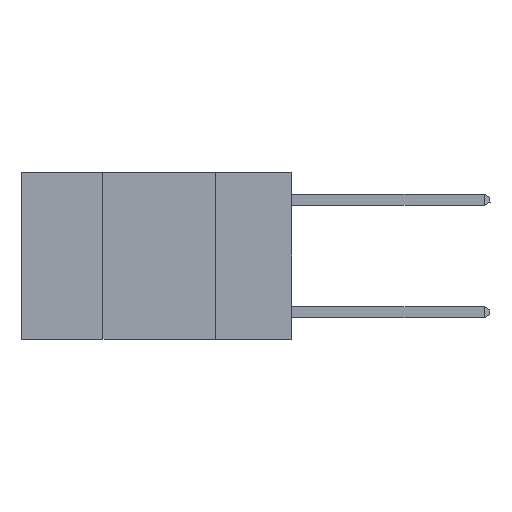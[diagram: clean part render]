
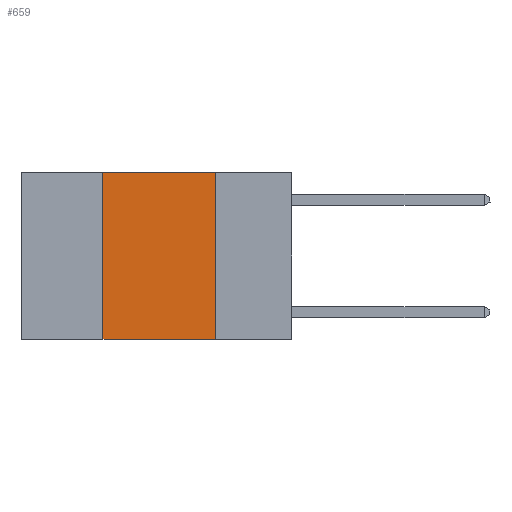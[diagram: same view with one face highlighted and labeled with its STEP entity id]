
A CAD part, left-side view. The second image highlights one B-rep face of the part: STEP entity #659.
In plain terms, the highlighted planar face has unit normal (-1, 0, 0).
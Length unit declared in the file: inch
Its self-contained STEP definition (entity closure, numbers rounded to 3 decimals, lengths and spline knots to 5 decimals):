
#45 = EDGE_LOOP ( 'NONE', ( #8960, #405, #11624, #4303 ) ) ;
#271 = VECTOR ( 'NONE', #1170, 39.37008 ) ;
#405 = ORIENTED_EDGE ( 'NONE', *, *, #2598, .F. ) ;
#479 = CARTESIAN_POINT ( 'NONE',  ( 0., 0.42, 0. ) ) ;
#531 = DIRECTION ( 'NONE',  ( 0., 0., 1. ) ) ;
#659 = ADVANCED_FACE ( 'NONE', ( #1397 ), #11835, .F. ) ;
#1170 = DIRECTION ( 'NONE',  ( 0., 0., -1. ) ) ;
#1397 = FACE_OUTER_BOUND ( 'NONE', #45, .T. ) ;
#1494 = DIRECTION ( 'NONE',  ( 0., -1., 0. ) ) ;
#1656 = CARTESIAN_POINT ( 'NONE',  ( 0., 0.6, -0.37 ) ) ;
#1747 = EDGE_CURVE ( 'NONE', #2354, #3298, #9297, .T. ) ;
#1871 = LINE ( 'NONE', #1656, #11259 ) ;
#2224 = CARTESIAN_POINT ( 'NONE',  ( 0., 0.17, -0.37 ) ) ;
#2354 = VERTEX_POINT ( 'NONE', #5978 ) ;
#2598 = EDGE_CURVE ( 'NONE', #3298, #3475, #3741, .T. ) ;
#3050 = LINE ( 'NONE', #6753, #271 ) ;
#3298 = VERTEX_POINT ( 'NONE', #8637 ) ;
#3448 = CARTESIAN_POINT ( 'NONE',  ( 0., 0.6, 0. ) ) ;
#3475 = VERTEX_POINT ( 'NONE', #5948 ) ;
#3714 = DIRECTION ( 'NONE',  ( 0., 0., -1. ) ) ;
#3741 = LINE ( 'NONE', #3955, #5592 ) ;
#3877 = DIRECTION ( 'NONE',  ( 0., -1., 0. ) ) ;
#3955 = CARTESIAN_POINT ( 'NONE',  ( 0., 0.6, 0. ) ) ;
#4303 = ORIENTED_EDGE ( 'NONE', *, *, #5254, .T. ) ;
#4455 = VECTOR ( 'NONE', #531, 39.37008 ) ;
#5254 = EDGE_CURVE ( 'NONE', #2354, #8116, #1871, .T. ) ;
#5592 = VECTOR ( 'NONE', #3877, 39.37008 ) ;
#5948 = CARTESIAN_POINT ( 'NONE',  ( 0., 0.17, 0. ) ) ;
#5978 = CARTESIAN_POINT ( 'NONE',  ( 0., 0.42, -0.37 ) ) ;
#6465 = DIRECTION ( 'NONE',  ( 1., 0., 0. ) ) ;
#6753 = CARTESIAN_POINT ( 'NONE',  ( 0., 0.17, 0. ) ) ;
#8116 = VERTEX_POINT ( 'NONE', #2224 ) ;
#8129 = EDGE_CURVE ( 'NONE', #3475, #8116, #3050, .T. ) ;
#8637 = CARTESIAN_POINT ( 'NONE',  ( 0., 0.42, 0. ) ) ;
#8960 = ORIENTED_EDGE ( 'NONE', *, *, #8129, .F. ) ;
#9297 = LINE ( 'NONE', #479, #4455 ) ;
#11003 = AXIS2_PLACEMENT_3D ( 'NONE', #3448, #6465, #3714 ) ;
#11259 = VECTOR ( 'NONE', #1494, 39.37008 ) ;
#11624 = ORIENTED_EDGE ( 'NONE', *, *, #1747, .F. ) ;
#11835 = PLANE ( 'NONE',  #11003 ) ;
